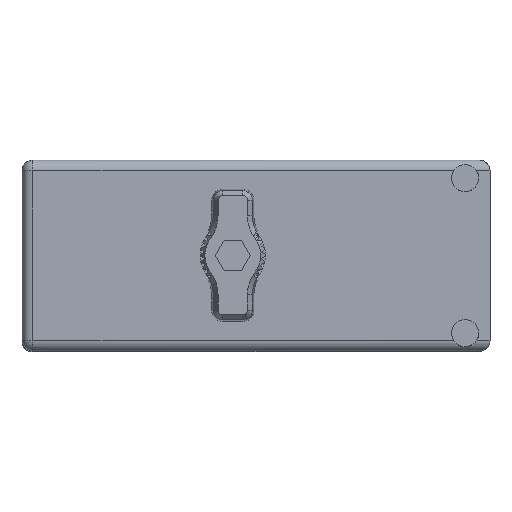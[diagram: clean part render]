
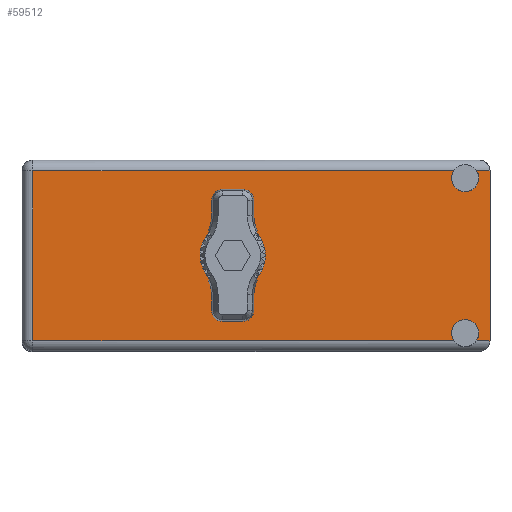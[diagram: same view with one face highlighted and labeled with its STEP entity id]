
A CAD part, top view. The second image highlights one B-rep face of the part: STEP entity #59512.
In plain terms, the highlighted face is planar.
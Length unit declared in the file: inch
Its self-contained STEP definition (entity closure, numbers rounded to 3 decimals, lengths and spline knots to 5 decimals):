
#4351 = VERTEX_POINT ( 'NONE', #37565 ) ;
#6104 = CARTESIAN_POINT ( 'NONE',  ( 1.659, 1.675, -0.547 ) ) ;
#6185 = DIRECTION ( 'NONE',  ( -1., 0., 0. ) ) ;
#6209 = CARTESIAN_POINT ( 'NONE',  ( 0., 1.675, 0. ) ) ;
#7143 = EDGE_CURVE ( 'NONE', #16013, #66157, #77677, .T. ) ;
#7982 = CARTESIAN_POINT ( 'NONE',  ( 1.499, 1.675, 0.5 ) ) ;
#9715 = VECTOR ( 'NONE', #50940, 39.37008 ) ;
#10744 = CIRCLE ( 'NONE', #37512, 0.0875 ) ;
#11545 = VERTEX_POINT ( 'NONE', #64320 ) ;
#11624 = LINE ( 'NONE', #51185, #40906 ) ;
#12121 = CARTESIAN_POINT ( 'NONE',  ( 1.499, 1.675, 0.5 ) ) ;
#12252 = DIRECTION ( 'NONE',  ( 0., 1., 0. ) ) ;
#12270 = ORIENTED_EDGE ( 'NONE', *, *, #72767, .T. ) ;
#12272 = CARTESIAN_POINT ( 'NONE',  ( -1.289, 1.675, -0.617 ) ) ;
#13059 = ORIENTED_EDGE ( 'NONE', *, *, #42772, .F. ) ;
#13153 = EDGE_CURVE ( 'NONE', #50779, #75017, #41271, .T. ) ;
#13246 = EDGE_CURVE ( 'NONE', #42276, #59518, #18876, .T. ) ;
#16013 = VERTEX_POINT ( 'NONE', #54687 ) ;
#18876 = LINE ( 'NONE', #28791, #31591 ) ;
#19347 = DIRECTION ( 'NONE',  ( 0., 1., 0. ) ) ;
#19396 = AXIS2_PLACEMENT_3D ( 'NONE', #12121, #55063, #42419 ) ;
#19522 = ORIENTED_EDGE ( 'NONE', *, *, #13246, .T. ) ;
#19603 = DIRECTION ( 'NONE',  ( 0., 1., 0. ) ) ;
#20282 = DIRECTION ( 'NONE',  ( -1., 0., 0. ) ) ;
#20554 = CARTESIAN_POINT ( 'NONE',  ( -1.359, 1.675, -0.547 ) ) ;
#21325 = DIRECTION ( 'NONE',  ( 0., 0., 1. ) ) ;
#21675 = LINE ( 'NONE', #12272, #64704 ) ;
#23248 = CARTESIAN_POINT ( 'NONE',  ( 0., 1.675, 0.125 ) ) ;
#23797 = DIRECTION ( 'NONE',  ( 0., 0., 1. ) ) ;
#25924 = DIRECTION ( 'NONE',  ( 0., 0., 1. ) ) ;
#26694 = VERTEX_POINT ( 'NONE', #50773 ) ;
#27345 = CARTESIAN_POINT ( 'NONE',  ( 1.659, 1.675, 0.617 ) ) ;
#27524 = VERTEX_POINT ( 'NONE', #23248 ) ;
#28791 = CARTESIAN_POINT ( 'NONE',  ( -1.359, 1.675, -0.547 ) ) ;
#28832 = CARTESIAN_POINT ( 'NONE',  ( 0., 1.675, 0. ) ) ;
#30863 = CARTESIAN_POINT ( 'NONE',  ( -1.359, 1.675, -0.617 ) ) ;
#31408 = DIRECTION ( 'NONE',  ( 0., 0., 1. ) ) ;
#31477 = EDGE_CURVE ( 'NONE', #75017, #11545, #21675, .T. ) ;
#31502 = EDGE_CURVE ( 'NONE', #69765, #27524, #50971, .T. ) ;
#31591 = VECTOR ( 'NONE', #35057, 39.37008 ) ;
#31759 = LINE ( 'NONE', #27345, #67943 ) ;
#32870 = ORIENTED_EDGE ( 'NONE', *, *, #55338, .F. ) ;
#33932 = EDGE_CURVE ( 'NONE', #66157, #4351, #35097, .T. ) ;
#35057 = DIRECTION ( 'NONE',  ( -1., 0., 0. ) ) ;
#35097 = CIRCLE ( 'NONE', #65411, 0.0875 ) ;
#36546 = ORIENTED_EDGE ( 'NONE', *, *, #31502, .F. ) ;
#37512 = AXIS2_PLACEMENT_3D ( 'NONE', #53844, #78140, #65858 ) ;
#37565 = CARTESIAN_POINT ( 'NONE',  ( 1.42519, 1.675, 0.547 ) ) ;
#38110 = DIRECTION ( 'NONE',  ( 0., 0., 1. ) ) ;
#38370 = VECTOR ( 'NONE', #20282, 39.37008 ) ;
#40634 = ORIENTED_EDGE ( 'NONE', *, *, #31477, .T. ) ;
#40906 = VECTOR ( 'NONE', #63768, 39.37008 ) ;
#41271 = LINE ( 'NONE', #20554, #38370 ) ;
#41587 = DIRECTION ( 'NONE',  ( 0., 0., 1. ) ) ;
#42276 = VERTEX_POINT ( 'NONE', #6104 ) ;
#42419 = DIRECTION ( 'NONE',  ( 0., 0., 1. ) ) ;
#42551 = CARTESIAN_POINT ( 'NONE',  ( 1.57281, 1.675, -0.547 ) ) ;
#42772 = EDGE_CURVE ( 'NONE', #27524, #69765, #48097, .T. ) ;
#45317 = EDGE_CURVE ( 'NONE', #42276, #26694, #31759, .T. ) ;
#45602 = ORIENTED_EDGE ( 'NONE', *, *, #7143, .F. ) ;
#46313 = FACE_OUTER_BOUND ( 'NONE', #47849, .T. ) ;
#47849 = EDGE_LOOP ( 'NONE', ( #50163, #78160, #45602, #12270, #58080, #19522, #51836, #32870, #58281, #40634 ) ) ;
#48097 = CIRCLE ( 'NONE', #71635, 0.125 ) ;
#49490 = EDGE_CURVE ( 'NONE', #11545, #4351, #11624, .T. ) ;
#50133 = CARTESIAN_POINT ( 'NONE',  ( 1.659, 1.675, 0.547 ) ) ;
#50163 = ORIENTED_EDGE ( 'NONE', *, *, #49490, .T. ) ;
#50773 = CARTESIAN_POINT ( 'NONE',  ( 1.659, 1.675, 0.547 ) ) ;
#50779 = VERTEX_POINT ( 'NONE', #71999 ) ;
#50940 = DIRECTION ( 'NONE',  ( 1., 0., 0. ) ) ;
#50971 = CIRCLE ( 'NONE', #64194, 0.125 ) ;
#51185 = CARTESIAN_POINT ( 'NONE',  ( 1.659, 1.675, 0.547 ) ) ;
#51474 = EDGE_CURVE ( 'NONE', #62966, #59518, #10744, .T. ) ;
#51836 = ORIENTED_EDGE ( 'NONE', *, *, #51474, .F. ) ;
#53844 = CARTESIAN_POINT ( 'NONE',  ( 1.499, 1.675, -0.5 ) ) ;
#54433 = EDGE_LOOP ( 'NONE', ( #13059, #36546 ) ) ;
#54687 = CARTESIAN_POINT ( 'NONE',  ( 1.57281, 1.675, 0.547 ) ) ;
#54771 = LINE ( 'NONE', #50133, #9715 ) ;
#55063 = DIRECTION ( 'NONE',  ( 0., 1., 0. ) ) ;
#55176 = CIRCLE ( 'NONE', #56677, 0.0875 ) ;
#55338 = EDGE_CURVE ( 'NONE', #50779, #62966, #55176, .T. ) ;
#55481 = CARTESIAN_POINT ( 'NONE',  ( 1.499, 1.675, -0.4125 ) ) ;
#55729 = PLANE ( 'NONE',  #73047 ) ;
#56677 = AXIS2_PLACEMENT_3D ( 'NONE', #69122, #19603, #31408 ) ;
#58080 = ORIENTED_EDGE ( 'NONE', *, *, #45317, .F. ) ;
#58281 = ORIENTED_EDGE ( 'NONE', *, *, #13153, .T. ) ;
#59073 = CARTESIAN_POINT ( 'NONE',  ( 1.499, 1.675, 0.4125 ) ) ;
#59512 = ADVANCED_FACE ( 'NONE', ( #62981, #46313 ), #55729, .T. ) ;
#59518 = VERTEX_POINT ( 'NONE', #42551 ) ;
#62966 = VERTEX_POINT ( 'NONE', #55481 ) ;
#62981 = FACE_BOUND ( 'NONE', #54433, .T. ) ;
#63768 = DIRECTION ( 'NONE',  ( 1., 0., 0. ) ) ;
#64194 = AXIS2_PLACEMENT_3D ( 'NONE', #6209, #19347, #25924 ) ;
#64320 = CARTESIAN_POINT ( 'NONE',  ( -1.289, 1.675, 0.547 ) ) ;
#64704 = VECTOR ( 'NONE', #23797, 39.37008 ) ;
#65411 = AXIS2_PLACEMENT_3D ( 'NONE', #7982, #69310, #38110 ) ;
#65858 = DIRECTION ( 'NONE',  ( 0., 0., 1. ) ) ;
#66157 = VERTEX_POINT ( 'NONE', #59073 ) ;
#67943 = VECTOR ( 'NONE', #21325, 39.37008 ) ;
#69122 = CARTESIAN_POINT ( 'NONE',  ( 1.499, 1.675, -0.5 ) ) ;
#69310 = DIRECTION ( 'NONE',  ( 0., 1., 0. ) ) ;
#69765 = VERTEX_POINT ( 'NONE', #76016 ) ;
#71635 = AXIS2_PLACEMENT_3D ( 'NONE', #28832, #72489, #41587 ) ;
#71999 = CARTESIAN_POINT ( 'NONE',  ( 1.42519, 1.675, -0.547 ) ) ;
#72489 = DIRECTION ( 'NONE',  ( 0., 1., 0. ) ) ;
#72521 = CARTESIAN_POINT ( 'NONE',  ( -1.289, 1.675, -0.547 ) ) ;
#72767 = EDGE_CURVE ( 'NONE', #16013, #26694, #54771, .T. ) ;
#73047 = AXIS2_PLACEMENT_3D ( 'NONE', #30863, #12252, #6185 ) ;
#75017 = VERTEX_POINT ( 'NONE', #72521 ) ;
#76016 = CARTESIAN_POINT ( 'NONE',  ( 0., 1.675, -0.125 ) ) ;
#77677 = CIRCLE ( 'NONE', #19396, 0.0875 ) ;
#78140 = DIRECTION ( 'NONE',  ( 0., 1., 0. ) ) ;
#78160 = ORIENTED_EDGE ( 'NONE', *, *, #33932, .F. ) ;
